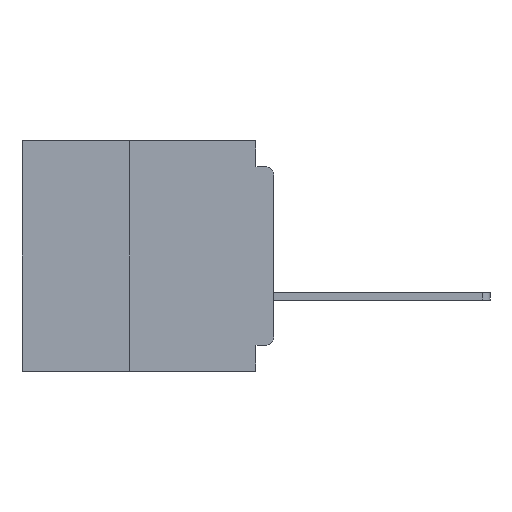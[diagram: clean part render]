
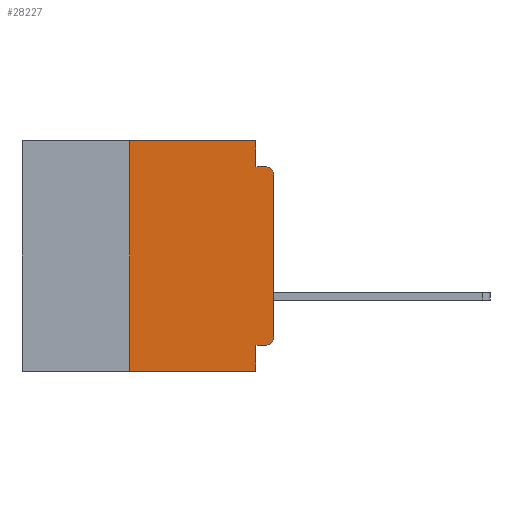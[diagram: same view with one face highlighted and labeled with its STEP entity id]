
A CAD part, left-side view. The second image highlights one B-rep face of the part: STEP entity #28227.
In plain terms, the highlighted planar face has unit normal (-1, 0, 0).
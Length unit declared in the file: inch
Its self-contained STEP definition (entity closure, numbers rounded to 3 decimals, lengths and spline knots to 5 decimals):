
#843 = DIRECTION ( 'NONE',  ( 1., 0., 0. ) ) ;
#1621 = EDGE_CURVE ( 'NONE', #49609, #2797, #13692, .T. ) ;
#2212 = CIRCLE ( 'NONE', #63488, 0.015 ) ;
#2797 = VERTEX_POINT ( 'NONE', #29401 ) ;
#3172 = EDGE_CURVE ( 'NONE', #41209, #42178, #51725, .T. ) ;
#6929 = VECTOR ( 'NONE', #9993, 39.37008 ) ;
#8014 = ORIENTED_EDGE ( 'NONE', *, *, #50510, .F. ) ;
#8448 = ORIENTED_EDGE ( 'NONE', *, *, #25257, .T. ) ;
#8470 = LINE ( 'NONE', #49166, #6929 ) ;
#8929 = CARTESIAN_POINT ( 'NONE',  ( 0., 0.031, -0.4 ) ) ;
#9020 = CARTESIAN_POINT ( 'NONE',  ( 0., 0.031, -0.355 ) ) ;
#9835 = EDGE_LOOP ( 'NONE', ( #42750, #58963, #8014, #33497, #26996, #13009, #56686, #11426, #10075, #8448 ) ) ;
#9864 = VECTOR ( 'NONE', #35005, 39.37008 ) ;
#9993 = DIRECTION ( 'NONE',  ( 0., 0., 1. ) ) ;
#10075 = ORIENTED_EDGE ( 'NONE', *, *, #33754, .F. ) ;
#10263 = VERTEX_POINT ( 'NONE', #46056 ) ;
#10564 = CARTESIAN_POINT ( 'NONE',  ( 0., 0.015, -0.045 ) ) ;
#11426 = ORIENTED_EDGE ( 'NONE', *, *, #1621, .F. ) ;
#13009 = ORIENTED_EDGE ( 'NONE', *, *, #51090, .F. ) ;
#13692 = LINE ( 'NONE', #8929, #15236 ) ;
#13864 = VECTOR ( 'NONE', #60454, 39.37008 ) ;
#13990 = VERTEX_POINT ( 'NONE', #51984 ) ;
#14404 = AXIS2_PLACEMENT_3D ( 'NONE', #53952, #24705, #58828 ) ;
#14432 = VECTOR ( 'NONE', #53838, 39.37008 ) ;
#14443 = CIRCLE ( 'NONE', #14404, 0.015 ) ;
#14855 = LINE ( 'NONE', #43605, #55332 ) ;
#14859 = EDGE_CURVE ( 'NONE', #42178, #13990, #14855, .T. ) ;
#15236 = VECTOR ( 'NONE', #34727, 39.37008 ) ;
#16040 = DIRECTION ( 'NONE',  ( -1., 0., 0. ) ) ;
#16259 = CARTESIAN_POINT ( 'NONE',  ( 0., 0.25, -0.4 ) ) ;
#18404 = CARTESIAN_POINT ( 'NONE',  ( 0., 0., -0.34 ) ) ;
#18420 = CARTESIAN_POINT ( 'NONE',  ( 0., 0.437, 0. ) ) ;
#19176 = DIRECTION ( 'NONE',  ( 0., 0., -1. ) ) ;
#20875 = VERTEX_POINT ( 'NONE', #18404 ) ;
#21164 = DIRECTION ( 'NONE',  ( 0., 0., 1. ) ) ;
#23334 = DIRECTION ( 'NONE',  ( 0., -1., 0. ) ) ;
#24705 = DIRECTION ( 'NONE',  ( -1., 0., 0. ) ) ;
#25257 = EDGE_CURVE ( 'NONE', #10263, #20875, #14443, .T. ) ;
#26140 = CARTESIAN_POINT ( 'NONE',  ( 0., 0., -0.045 ) ) ;
#26931 = VERTEX_POINT ( 'NONE', #10564 ) ;
#26996 = ORIENTED_EDGE ( 'NONE', *, *, #3172, .F. ) ;
#27458 = LINE ( 'NONE', #58711, #14432 ) ;
#28227 = ADVANCED_FACE ( 'NONE', ( #51386 ), #59566, .F. ) ;
#29401 = CARTESIAN_POINT ( 'NONE',  ( 0., 0.031, -0.4 ) ) ;
#29975 = EDGE_CURVE ( 'NONE', #58324, #2797, #35991, .T. ) ;
#33497 = ORIENTED_EDGE ( 'NONE', *, *, #14859, .F. ) ;
#33731 = LINE ( 'NONE', #16259, #55033 ) ;
#33754 = EDGE_CURVE ( 'NONE', #10263, #49609, #27458, .T. ) ;
#34727 = DIRECTION ( 'NONE',  ( 0., 0., -1. ) ) ;
#35005 = DIRECTION ( 'NONE',  ( 0., -1., 0. ) ) ;
#35329 = DIRECTION ( 'NONE',  ( 0., 0., -1. ) ) ;
#35991 = LINE ( 'NONE', #39930, #9864 ) ;
#38457 = VERTEX_POINT ( 'NONE', #54110 ) ;
#39217 = AXIS2_PLACEMENT_3D ( 'NONE', #44930, #843, #35329 ) ;
#39930 = CARTESIAN_POINT ( 'NONE',  ( 0., 0.437, -0.4 ) ) ;
#39947 = LINE ( 'NONE', #26140, #13864 ) ;
#41209 = VERTEX_POINT ( 'NONE', #54612 ) ;
#42178 = VERTEX_POINT ( 'NONE', #47268 ) ;
#42572 = EDGE_CURVE ( 'NONE', #38457, #26931, #2212, .T. ) ;
#42750 = ORIENTED_EDGE ( 'NONE', *, *, #47913, .T. ) ;
#43605 = CARTESIAN_POINT ( 'NONE',  ( 0., 0.031, 0. ) ) ;
#44930 = CARTESIAN_POINT ( 'NONE',  ( 0., 0.437, 0. ) ) ;
#45330 = CARTESIAN_POINT ( 'NONE',  ( 0., 0.015, -0.06 ) ) ;
#46056 = CARTESIAN_POINT ( 'NONE',  ( 0., 0.015, -0.355 ) ) ;
#47268 = CARTESIAN_POINT ( 'NONE',  ( 0., 0.031, 0. ) ) ;
#47913 = EDGE_CURVE ( 'NONE', #20875, #38457, #8470, .T. ) ;
#49166 = CARTESIAN_POINT ( 'NONE',  ( 0., 0., 0. ) ) ;
#49609 = VERTEX_POINT ( 'NONE', #9020 ) ;
#50182 = VECTOR ( 'NONE', #23334, 39.37008 ) ;
#50199 = DIRECTION ( 'NONE',  ( 0., 0., -1. ) ) ;
#50510 = EDGE_CURVE ( 'NONE', #13990, #26931, #39947, .T. ) ;
#51090 = EDGE_CURVE ( 'NONE', #58324, #41209, #33731, .T. ) ;
#51386 = FACE_OUTER_BOUND ( 'NONE', #9835, .T. ) ;
#51725 = LINE ( 'NONE', #18420, #50182 ) ;
#51984 = CARTESIAN_POINT ( 'NONE',  ( 0., 0.031, -0.045 ) ) ;
#53838 = DIRECTION ( 'NONE',  ( 0., 1., 0. ) ) ;
#53952 = CARTESIAN_POINT ( 'NONE',  ( 0., 0.015, -0.34 ) ) ;
#54110 = CARTESIAN_POINT ( 'NONE',  ( 0., 0., -0.06 ) ) ;
#54241 = CARTESIAN_POINT ( 'NONE',  ( 0., 0.25, -0.4 ) ) ;
#54612 = CARTESIAN_POINT ( 'NONE',  ( 0., 0.25, 0. ) ) ;
#55033 = VECTOR ( 'NONE', #21164, 39.37008 ) ;
#55332 = VECTOR ( 'NONE', #19176, 39.37008 ) ;
#56686 = ORIENTED_EDGE ( 'NONE', *, *, #29975, .T. ) ;
#58324 = VERTEX_POINT ( 'NONE', #54241 ) ;
#58711 = CARTESIAN_POINT ( 'NONE',  ( 0., 0., -0.355 ) ) ;
#58828 = DIRECTION ( 'NONE',  ( 0., 0., -1. ) ) ;
#58963 = ORIENTED_EDGE ( 'NONE', *, *, #42572, .T. ) ;
#59566 = PLANE ( 'NONE',  #39217 ) ;
#60454 = DIRECTION ( 'NONE',  ( 0., -1., 0. ) ) ;
#63488 = AXIS2_PLACEMENT_3D ( 'NONE', #45330, #16040, #50199 ) ;
